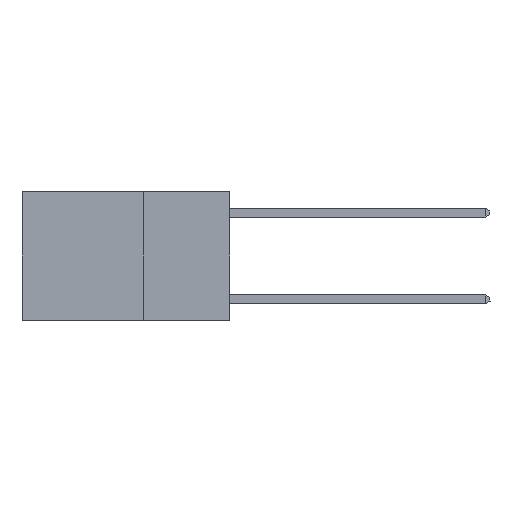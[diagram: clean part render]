
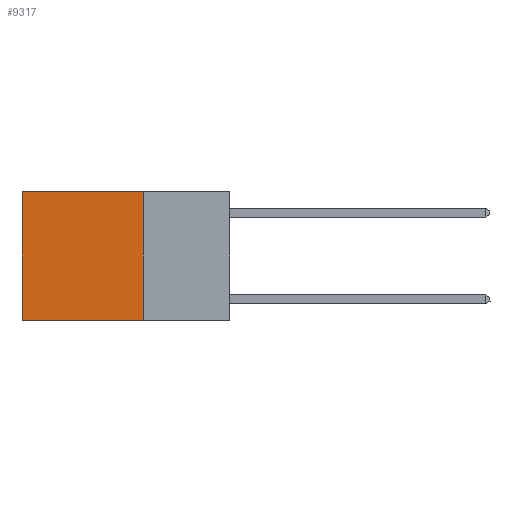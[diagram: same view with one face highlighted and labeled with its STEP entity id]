
A CAD part, left-side view. The second image highlights one B-rep face of the part: STEP entity #9317.
In plain terms, the highlighted planar face has unit normal (-1, 0, 0).
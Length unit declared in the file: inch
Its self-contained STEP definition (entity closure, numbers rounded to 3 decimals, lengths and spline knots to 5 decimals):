
#743 = EDGE_CURVE ( 'NONE', #2359, #12996, #9319, .T. ) ;
#1095 = VECTOR ( 'NONE', #21058, 39.37008 ) ;
#2359 = VERTEX_POINT ( 'NONE', #3464 ) ;
#3258 = DIRECTION ( 'NONE',  ( 1., 0., 0. ) ) ;
#3464 = CARTESIAN_POINT ( 'NONE',  ( 0.2625, 0.25, 0. ) ) ;
#4798 = PLANE ( 'NONE',  #12688 ) ;
#5896 = EDGE_CURVE ( 'NONE', #12996, #19467, #13491, .T. ) ;
#5971 = EDGE_CURVE ( 'NONE', #2359, #19678, #12942, .T. ) ;
#6106 = DIRECTION ( 'NONE',  ( 0., 1., 0. ) ) ;
#6806 = EDGE_LOOP ( 'NONE', ( #16534, #17748, #8006, #11270 ) ) ;
#7352 = CARTESIAN_POINT ( 'NONE',  ( 0.2625, 0.25, -0.37 ) ) ;
#8006 = ORIENTED_EDGE ( 'NONE', *, *, #5971, .F. ) ;
#8390 = DIRECTION ( 'NONE',  ( 0., 0., -1. ) ) ;
#9317 = ADVANCED_FACE ( 'NONE', ( #16723 ), #4798, .F. ) ;
#9319 = LINE ( 'NONE', #9967, #18617 ) ;
#9967 = CARTESIAN_POINT ( 'NONE',  ( 0.2625, 0.25, 0. ) ) ;
#10067 = DIRECTION ( 'NONE',  ( 0., 0., -1. ) ) ;
#10530 = CARTESIAN_POINT ( 'NONE',  ( 0.2625, 0.6, -0.37 ) ) ;
#11032 = DIRECTION ( 'NONE',  ( 0., 1., 0. ) ) ;
#11270 = ORIENTED_EDGE ( 'NONE', *, *, #743, .T. ) ;
#12682 = EDGE_CURVE ( 'NONE', #19678, #19467, #13849, .T. ) ;
#12688 = AXIS2_PLACEMENT_3D ( 'NONE', #13802, #3258, #10067 ) ;
#12942 = LINE ( 'NONE', #15901, #1095 ) ;
#12996 = VERTEX_POINT ( 'NONE', #17518 ) ;
#13491 = LINE ( 'NONE', #13768, #19810 ) ;
#13768 = CARTESIAN_POINT ( 'NONE',  ( 0.2625, 0.6, 0. ) ) ;
#13802 = CARTESIAN_POINT ( 'NONE',  ( 0.2625, 0.25, 0. ) ) ;
#13849 = LINE ( 'NONE', #18128, #17139 ) ;
#15901 = CARTESIAN_POINT ( 'NONE',  ( 0.2625, 0.25, 0. ) ) ;
#16534 = ORIENTED_EDGE ( 'NONE', *, *, #5896, .T. ) ;
#16723 = FACE_OUTER_BOUND ( 'NONE', #6806, .T. ) ;
#17139 = VECTOR ( 'NONE', #11032, 39.37008 ) ;
#17518 = CARTESIAN_POINT ( 'NONE',  ( 0.2625, 0.6, 0. ) ) ;
#17748 = ORIENTED_EDGE ( 'NONE', *, *, #12682, .F. ) ;
#18128 = CARTESIAN_POINT ( 'NONE',  ( 0.2625, 0.25, -0.37 ) ) ;
#18617 = VECTOR ( 'NONE', #6106, 39.37008 ) ;
#19467 = VERTEX_POINT ( 'NONE', #10530 ) ;
#19678 = VERTEX_POINT ( 'NONE', #7352 ) ;
#19810 = VECTOR ( 'NONE', #8390, 39.37008 ) ;
#21058 = DIRECTION ( 'NONE',  ( 0., 0., -1. ) ) ;
